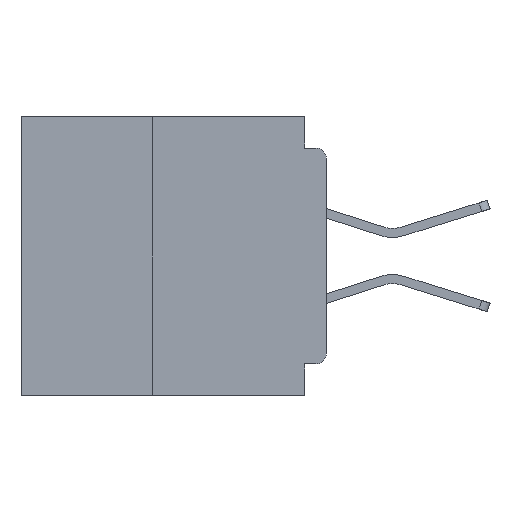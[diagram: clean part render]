
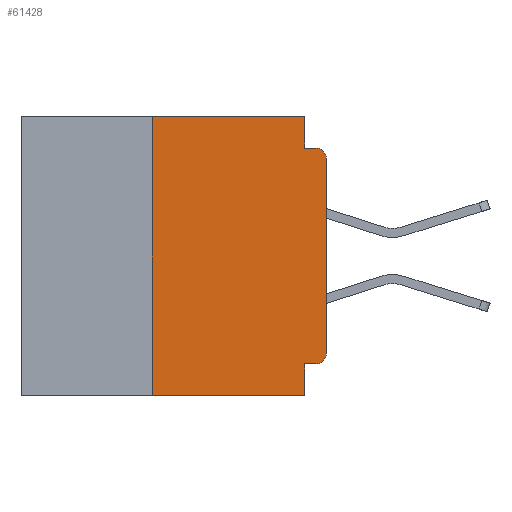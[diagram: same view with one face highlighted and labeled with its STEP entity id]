
A CAD part, left-side view. The second image highlights one B-rep face of the part: STEP entity #61428.
In plain terms, the highlighted planar face has unit normal (-1, 0, 0).
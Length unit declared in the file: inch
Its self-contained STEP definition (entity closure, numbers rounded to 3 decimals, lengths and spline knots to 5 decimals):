
#908 = VERTEX_POINT ( 'NONE', #49245 ) ;
#1125 = CARTESIAN_POINT ( 'NONE',  ( 0., 0.015, -0.045 ) ) ;
#1444 = VECTOR ( 'NONE', #54648, 39.37008 ) ;
#2331 = CARTESIAN_POINT ( 'NONE',  ( 0., 0., -0.06 ) ) ;
#3220 = DIRECTION ( 'NONE',  ( 0., 0., -1. ) ) ;
#3432 = DIRECTION ( 'NONE',  ( 0., 0., -1. ) ) ;
#4112 = EDGE_CURVE ( 'NONE', #17826, #37282, #36839, .T. ) ;
#4832 = DIRECTION ( 'NONE',  ( 0., 0., -1. ) ) ;
#4898 = ORIENTED_EDGE ( 'NONE', *, *, #61485, .F. ) ;
#5597 = VERTEX_POINT ( 'NONE', #19852 ) ;
#6035 = VERTEX_POINT ( 'NONE', #60662 ) ;
#6673 = EDGE_CURVE ( 'NONE', #56217, #52838, #23123, .T. ) ;
#7335 = CARTESIAN_POINT ( 'NONE',  ( 0., 0., -0.045 ) ) ;
#10253 = VERTEX_POINT ( 'NONE', #32841 ) ;
#11350 = AXIS2_PLACEMENT_3D ( 'NONE', #45949, #31814, #3220 ) ;
#11603 = EDGE_LOOP ( 'NONE', ( #48870, #12295, #50356, #16815, #31027, #48140, #24332, #28805, #4898, #58671 ) ) ;
#12295 = ORIENTED_EDGE ( 'NONE', *, *, #46933, .T. ) ;
#12644 = DIRECTION ( 'NONE',  ( 0., 0., 1. ) ) ;
#13994 = VECTOR ( 'NONE', #4832, 39.37008 ) ;
#14183 = CARTESIAN_POINT ( 'NONE',  ( 0., 0.031, 0. ) ) ;
#14860 = EDGE_CURVE ( 'NONE', #19108, #17826, #20102, .T. ) ;
#16815 = ORIENTED_EDGE ( 'NONE', *, *, #29998, .F. ) ;
#17393 = PLANE ( 'NONE',  #11350 ) ;
#17826 = VERTEX_POINT ( 'NONE', #59687 ) ;
#18746 = VECTOR ( 'NONE', #20545, 39.37008 ) ;
#19108 = VERTEX_POINT ( 'NONE', #21469 ) ;
#19852 = CARTESIAN_POINT ( 'NONE',  ( 0., 0.25, 0. ) ) ;
#20102 = CIRCLE ( 'NONE', #56539, 0.015 ) ;
#20545 = DIRECTION ( 'NONE',  ( 0., 0., 1. ) ) ;
#20580 = AXIS2_PLACEMENT_3D ( 'NONE', #55546, #26992, #60350 ) ;
#20626 = CARTESIAN_POINT ( 'NONE',  ( 0., 0.015, -0.34 ) ) ;
#21469 = CARTESIAN_POINT ( 'NONE',  ( 0., 0.015, -0.355 ) ) ;
#22630 = CARTESIAN_POINT ( 'NONE',  ( 0., 0., -0.355 ) ) ;
#23123 = LINE ( 'NONE', #36784, #35784 ) ;
#23351 = VECTOR ( 'NONE', #28116, 39.37008 ) ;
#23371 = LINE ( 'NONE', #26434, #47201 ) ;
#24151 = VERTEX_POINT ( 'NONE', #1125 ) ;
#24332 = ORIENTED_EDGE ( 'NONE', *, *, #39235, .T. ) ;
#25421 = DIRECTION ( 'NONE',  ( 0., 0., -1. ) ) ;
#26434 = CARTESIAN_POINT ( 'NONE',  ( 0., 0.437, 0. ) ) ;
#26847 = LINE ( 'NONE', #7335, #1444 ) ;
#26992 = DIRECTION ( 'NONE',  ( -1., 0., 0. ) ) ;
#28116 = DIRECTION ( 'NONE',  ( 0., -1., 0. ) ) ;
#28805 = ORIENTED_EDGE ( 'NONE', *, *, #6673, .F. ) ;
#29952 = LINE ( 'NONE', #44235, #18746 ) ;
#29998 = EDGE_CURVE ( 'NONE', #10253, #6035, #61780, .T. ) ;
#31027 = ORIENTED_EDGE ( 'NONE', *, *, #41502, .F. ) ;
#31814 = DIRECTION ( 'NONE',  ( 1., 0., 0. ) ) ;
#32841 = CARTESIAN_POINT ( 'NONE',  ( 0., 0.031, 0. ) ) ;
#34647 = EDGE_CURVE ( 'NONE', #6035, #24151, #26847, .T. ) ;
#35784 = VECTOR ( 'NONE', #3432, 39.37008 ) ;
#36395 = DIRECTION ( 'NONE',  ( 0., -1., 0. ) ) ;
#36784 = CARTESIAN_POINT ( 'NONE',  ( 0., 0.031, -0.4 ) ) ;
#36839 = LINE ( 'NONE', #50807, #60752 ) ;
#37282 = VERTEX_POINT ( 'NONE', #2331 ) ;
#38430 = CARTESIAN_POINT ( 'NONE',  ( 0., 0.031, -0.4 ) ) ;
#39235 = EDGE_CURVE ( 'NONE', #908, #52838, #61377, .T. ) ;
#41502 = EDGE_CURVE ( 'NONE', #5597, #10253, #23371, .T. ) ;
#44235 = CARTESIAN_POINT ( 'NONE',  ( 0., 0.25, -0.4 ) ) ;
#44532 = VECTOR ( 'NONE', #55973, 39.37008 ) ;
#45949 = CARTESIAN_POINT ( 'NONE',  ( 0., 0.437, 0. ) ) ;
#46042 = LINE ( 'NONE', #22630, #44532 ) ;
#46506 = CARTESIAN_POINT ( 'NONE',  ( 0., 0.031, -0.355 ) ) ;
#46933 = EDGE_CURVE ( 'NONE', #37282, #24151, #49891, .T. ) ;
#47059 = CARTESIAN_POINT ( 'NONE',  ( 0., 0.437, -0.4 ) ) ;
#47201 = VECTOR ( 'NONE', #36395, 39.37008 ) ;
#48140 = ORIENTED_EDGE ( 'NONE', *, *, #55912, .F. ) ;
#48870 = ORIENTED_EDGE ( 'NONE', *, *, #4112, .T. ) ;
#49245 = CARTESIAN_POINT ( 'NONE',  ( 0., 0.25, -0.4 ) ) ;
#49891 = CIRCLE ( 'NONE', #20580, 0.015 ) ;
#50356 = ORIENTED_EDGE ( 'NONE', *, *, #34647, .F. ) ;
#50807 = CARTESIAN_POINT ( 'NONE',  ( 0., 0., 0. ) ) ;
#52838 = VERTEX_POINT ( 'NONE', #38430 ) ;
#53922 = DIRECTION ( 'NONE',  ( -1., 0., 0. ) ) ;
#54648 = DIRECTION ( 'NONE',  ( 0., -1., 0. ) ) ;
#55546 = CARTESIAN_POINT ( 'NONE',  ( 0., 0.015, -0.06 ) ) ;
#55912 = EDGE_CURVE ( 'NONE', #908, #5597, #29952, .T. ) ;
#55973 = DIRECTION ( 'NONE',  ( 0., 1., 0. ) ) ;
#56217 = VERTEX_POINT ( 'NONE', #46506 ) ;
#56539 = AXIS2_PLACEMENT_3D ( 'NONE', #20626, #53922, #25421 ) ;
#58671 = ORIENTED_EDGE ( 'NONE', *, *, #14860, .T. ) ;
#58791 = FACE_OUTER_BOUND ( 'NONE', #11603, .T. ) ;
#59687 = CARTESIAN_POINT ( 'NONE',  ( 0., 0., -0.34 ) ) ;
#60350 = DIRECTION ( 'NONE',  ( 0., 0., -1. ) ) ;
#60662 = CARTESIAN_POINT ( 'NONE',  ( 0., 0.031, -0.045 ) ) ;
#60752 = VECTOR ( 'NONE', #12644, 39.37008 ) ;
#61377 = LINE ( 'NONE', #47059, #23351 ) ;
#61428 = ADVANCED_FACE ( 'NONE', ( #58791 ), #17393, .F. ) ;
#61485 = EDGE_CURVE ( 'NONE', #19108, #56217, #46042, .T. ) ;
#61780 = LINE ( 'NONE', #14183, #13994 ) ;
